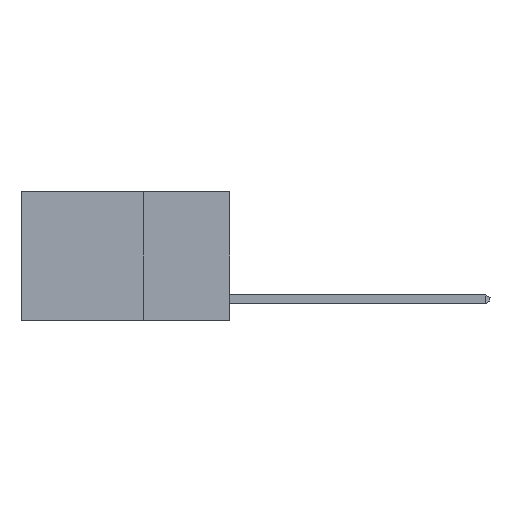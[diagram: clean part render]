
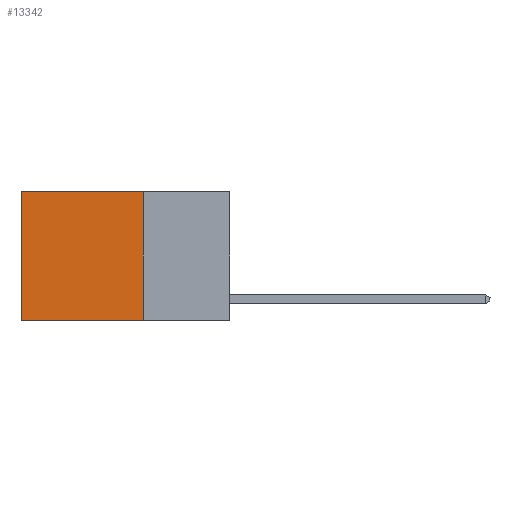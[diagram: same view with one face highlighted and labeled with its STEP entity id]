
A CAD part, left-side view. The second image highlights one B-rep face of the part: STEP entity #13342.
In plain terms, the highlighted planar face has unit normal (-1, 0, 0).
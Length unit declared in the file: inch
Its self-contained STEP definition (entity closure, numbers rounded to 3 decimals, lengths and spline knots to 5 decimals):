
#472 = LINE ( 'NONE', #617, #28483 ) ;
#513 = AXIS2_PLACEMENT_3D ( 'NONE', #30296, #1836, #6295 ) ;
#617 = CARTESIAN_POINT ( 'NONE',  ( 0.2625, 0.25, -0.37 ) ) ;
#1836 = DIRECTION ( 'NONE',  ( 1., 0., 0. ) ) ;
#3518 = EDGE_CURVE ( 'NONE', #18382, #25636, #10811, .T. ) ;
#4162 = PLANE ( 'NONE',  #513 ) ;
#5752 = VECTOR ( 'NONE', #8949, 39.37008 ) ;
#5782 = LINE ( 'NONE', #19649, #16426 ) ;
#6295 = DIRECTION ( 'NONE',  ( 0., 0., -1. ) ) ;
#6500 = VECTOR ( 'NONE', #27895, 39.37008 ) ;
#8221 = ORIENTED_EDGE ( 'NONE', *, *, #21474, .F. ) ;
#8949 = DIRECTION ( 'NONE',  ( 0., 1., 0. ) ) ;
#10417 = CARTESIAN_POINT ( 'NONE',  ( 0.2625, 0.6, -0.37 ) ) ;
#10650 = EDGE_LOOP ( 'NONE', ( #11737, #19759, #8221, #26946 ) ) ;
#10811 = LINE ( 'NONE', #25266, #5752 ) ;
#11100 = CARTESIAN_POINT ( 'NONE',  ( 0.2625, 0.6, 0. ) ) ;
#11461 = CARTESIAN_POINT ( 'NONE',  ( 0.2625, 0.6, 0. ) ) ;
#11737 = ORIENTED_EDGE ( 'NONE', *, *, #15418, .T. ) ;
#13342 = ADVANCED_FACE ( 'NONE', ( #20320 ), #4162, .F. ) ;
#15418 = EDGE_CURVE ( 'NONE', #25636, #27672, #27438, .T. ) ;
#16426 = VECTOR ( 'NONE', #24716, 39.37008 ) ;
#18382 = VERTEX_POINT ( 'NONE', #24967 ) ;
#19649 = CARTESIAN_POINT ( 'NONE',  ( 0.2625, 0.25, 0. ) ) ;
#19759 = ORIENTED_EDGE ( 'NONE', *, *, #29197, .F. ) ;
#20103 = CARTESIAN_POINT ( 'NONE',  ( 0.2625, 0.25, -0.37 ) ) ;
#20320 = FACE_OUTER_BOUND ( 'NONE', #10650, .T. ) ;
#21474 = EDGE_CURVE ( 'NONE', #18382, #27741, #5782, .T. ) ;
#24716 = DIRECTION ( 'NONE',  ( 0., 0., -1. ) ) ;
#24967 = CARTESIAN_POINT ( 'NONE',  ( 0.2625, 0.25, 0. ) ) ;
#25266 = CARTESIAN_POINT ( 'NONE',  ( 0.2625, 0.25, 0. ) ) ;
#25636 = VERTEX_POINT ( 'NONE', #11100 ) ;
#26946 = ORIENTED_EDGE ( 'NONE', *, *, #3518, .T. ) ;
#27438 = LINE ( 'NONE', #11461, #6500 ) ;
#27672 = VERTEX_POINT ( 'NONE', #10417 ) ;
#27741 = VERTEX_POINT ( 'NONE', #20103 ) ;
#27895 = DIRECTION ( 'NONE',  ( 0., 0., -1. ) ) ;
#28483 = VECTOR ( 'NONE', #28619, 39.37008 ) ;
#28619 = DIRECTION ( 'NONE',  ( 0., 1., 0. ) ) ;
#29197 = EDGE_CURVE ( 'NONE', #27741, #27672, #472, .T. ) ;
#30296 = CARTESIAN_POINT ( 'NONE',  ( 0.2625, 0.25, 0. ) ) ;
